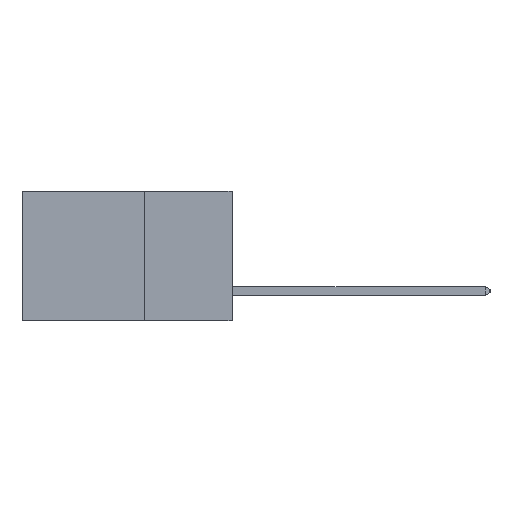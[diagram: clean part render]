
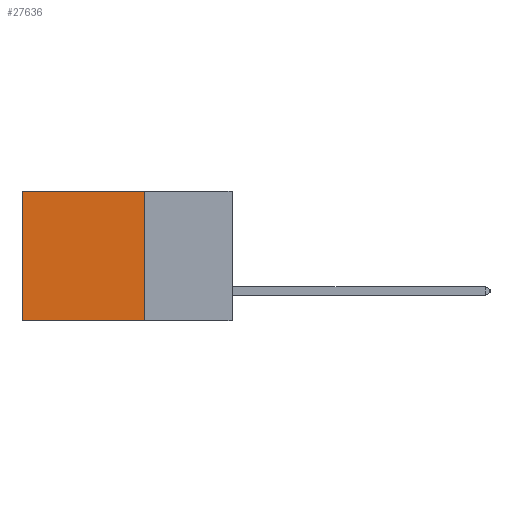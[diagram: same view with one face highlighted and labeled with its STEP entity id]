
A CAD part, left-side view. The second image highlights one B-rep face of the part: STEP entity #27636.
In plain terms, the highlighted planar face has unit normal (-1, 0, 0).
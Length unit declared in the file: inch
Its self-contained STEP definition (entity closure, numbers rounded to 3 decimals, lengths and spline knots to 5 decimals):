
#1595 = CARTESIAN_POINT ( 'NONE',  ( 0.2875, 0.25, 0. ) ) ;
#2182 = DIRECTION ( 'NONE',  ( 0., 0., -1. ) ) ;
#3926 = DIRECTION ( 'NONE',  ( 0., 0., -1. ) ) ;
#4047 = CARTESIAN_POINT ( 'NONE',  ( 0.2875, 0.25, -0.37 ) ) ;
#4382 = EDGE_LOOP ( 'NONE', ( #35446, #22018, #18502, #9916 ) ) ;
#6967 = DIRECTION ( 'NONE',  ( 0., 1., 0. ) ) ;
#8292 = EDGE_CURVE ( 'NONE', #30082, #29837, #19361, .T. ) ;
#9916 = ORIENTED_EDGE ( 'NONE', *, *, #23894, .T. ) ;
#10912 = CARTESIAN_POINT ( 'NONE',  ( 0.2875, 0.6, 0. ) ) ;
#11705 = VECTOR ( 'NONE', #6967, 39.37008 ) ;
#12371 = EDGE_CURVE ( 'NONE', #17077, #29837, #17135, .T. ) ;
#14819 = DIRECTION ( 'NONE',  ( 0., 0., -1. ) ) ;
#15523 = LINE ( 'NONE', #1595, #29718 ) ;
#17077 = VERTEX_POINT ( 'NONE', #35579 ) ;
#17135 = LINE ( 'NONE', #10912, #23811 ) ;
#18344 = CARTESIAN_POINT ( 'NONE',  ( 0.2875, 0.25, 0. ) ) ;
#18502 = ORIENTED_EDGE ( 'NONE', *, *, #19876, .F. ) ;
#19361 = LINE ( 'NONE', #4047, #11705 ) ;
#19876 = EDGE_CURVE ( 'NONE', #34448, #30082, #25741, .T. ) ;
#21170 = DIRECTION ( 'NONE',  ( 1., 0., 0. ) ) ;
#21757 = DIRECTION ( 'NONE',  ( 0., 1., 0. ) ) ;
#22018 = ORIENTED_EDGE ( 'NONE', *, *, #8292, .F. ) ;
#23811 = VECTOR ( 'NONE', #2182, 39.37008 ) ;
#23836 = CARTESIAN_POINT ( 'NONE',  ( 0.2875, 0.6, -0.37 ) ) ;
#23894 = EDGE_CURVE ( 'NONE', #34448, #17077, #15523, .T. ) ;
#24850 = VECTOR ( 'NONE', #14819, 39.37008 ) ;
#25741 = LINE ( 'NONE', #28942, #24850 ) ;
#27636 = ADVANCED_FACE ( 'NONE', ( #31164 ), #35165, .F. ) ;
#28942 = CARTESIAN_POINT ( 'NONE',  ( 0.2875, 0.25, 0. ) ) ;
#29535 = CARTESIAN_POINT ( 'NONE',  ( 0.2875, 0.25, 0. ) ) ;
#29718 = VECTOR ( 'NONE', #21757, 39.37008 ) ;
#29837 = VERTEX_POINT ( 'NONE', #23836 ) ;
#30082 = VERTEX_POINT ( 'NONE', #36552 ) ;
#31164 = FACE_OUTER_BOUND ( 'NONE', #4382, .T. ) ;
#32653 = AXIS2_PLACEMENT_3D ( 'NONE', #18344, #21170, #3926 ) ;
#34448 = VERTEX_POINT ( 'NONE', #29535 ) ;
#35165 = PLANE ( 'NONE',  #32653 ) ;
#35446 = ORIENTED_EDGE ( 'NONE', *, *, #12371, .T. ) ;
#35579 = CARTESIAN_POINT ( 'NONE',  ( 0.2875, 0.6, 0. ) ) ;
#36552 = CARTESIAN_POINT ( 'NONE',  ( 0.2875, 0.25, -0.37 ) ) ;
